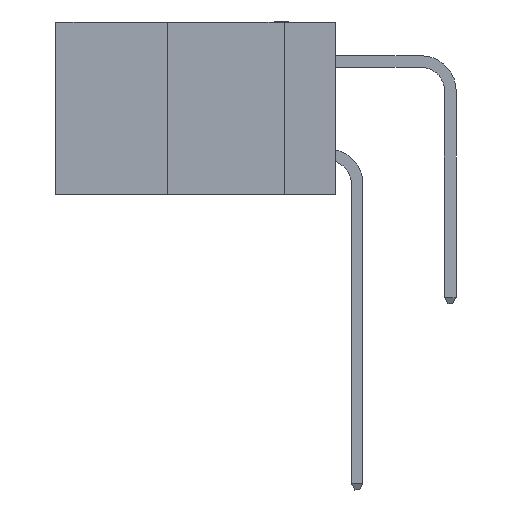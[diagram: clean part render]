
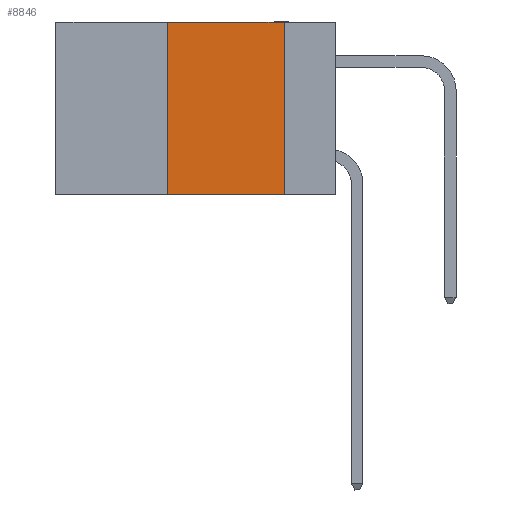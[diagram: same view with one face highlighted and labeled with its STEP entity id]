
A CAD part, left-side view. The second image highlights one B-rep face of the part: STEP entity #8846.
In plain terms, the highlighted planar face has unit normal (-1, 0, 0).
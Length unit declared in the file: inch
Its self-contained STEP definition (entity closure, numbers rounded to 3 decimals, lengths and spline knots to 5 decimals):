
#2086 = DIRECTION ( 'NONE',  ( 0., 0., -1. ) ) ;
#2624 = DIRECTION ( 'NONE',  ( 0., -1., 0. ) ) ;
#2887 = CARTESIAN_POINT ( 'NONE',  ( 0., 0.11, 0. ) ) ;
#3081 = VERTEX_POINT ( 'NONE', #8731 ) ;
#3131 = VECTOR ( 'NONE', #20635, 39.37008 ) ;
#3666 = ORIENTED_EDGE ( 'NONE', *, *, #10331, .F. ) ;
#5319 = ORIENTED_EDGE ( 'NONE', *, *, #9686, .T. ) ;
#6051 = CARTESIAN_POINT ( 'NONE',  ( 0., 0.6, -0.37 ) ) ;
#6799 = CARTESIAN_POINT ( 'NONE',  ( 0., 0.36, 0. ) ) ;
#7475 = DIRECTION ( 'NONE',  ( 0., 0., 1. ) ) ;
#8731 = CARTESIAN_POINT ( 'NONE',  ( 0., 0.11, 0. ) ) ;
#8846 = ADVANCED_FACE ( 'NONE', ( #18872 ), #16088, .F. ) ;
#9374 = LINE ( 'NONE', #6051, #3131 ) ;
#9686 = EDGE_CURVE ( 'NONE', #26777, #34970, #9374, .T. ) ;
#10331 = EDGE_CURVE ( 'NONE', #23102, #3081, #29275, .T. ) ;
#10421 = CARTESIAN_POINT ( 'NONE',  ( 0., 0.36, 0. ) ) ;
#10741 = DIRECTION ( 'NONE',  ( 1., 0., 0. ) ) ;
#13022 = CARTESIAN_POINT ( 'NONE',  ( 0., 0.36, -0.37 ) ) ;
#13854 = CARTESIAN_POINT ( 'NONE',  ( 0., 0.11, -0.37 ) ) ;
#16088 = PLANE ( 'NONE',  #21588 ) ;
#16873 = EDGE_LOOP ( 'NONE', ( #29009, #3666, #35339, #5319 ) ) ;
#18308 = EDGE_CURVE ( 'NONE', #26777, #23102, #31670, .T. ) ;
#18872 = FACE_OUTER_BOUND ( 'NONE', #16873, .T. ) ;
#19139 = VECTOR ( 'NONE', #2624, 39.37008 ) ;
#20635 = DIRECTION ( 'NONE',  ( 0., -1., 0. ) ) ;
#21588 = AXIS2_PLACEMENT_3D ( 'NONE', #27372, #10741, #2086 ) ;
#21931 = EDGE_CURVE ( 'NONE', #3081, #34970, #30224, .T. ) ;
#22438 = DIRECTION ( 'NONE',  ( 0., 0., -1. ) ) ;
#22921 = CARTESIAN_POINT ( 'NONE',  ( 0., 0.6, 0. ) ) ;
#23102 = VERTEX_POINT ( 'NONE', #6799 ) ;
#26744 = VECTOR ( 'NONE', #7475, 39.37008 ) ;
#26777 = VERTEX_POINT ( 'NONE', #13022 ) ;
#27372 = CARTESIAN_POINT ( 'NONE',  ( 0., 0.6, 0. ) ) ;
#29009 = ORIENTED_EDGE ( 'NONE', *, *, #21931, .F. ) ;
#29275 = LINE ( 'NONE', #22921, #19139 ) ;
#30224 = LINE ( 'NONE', #2887, #33942 ) ;
#31670 = LINE ( 'NONE', #10421, #26744 ) ;
#33942 = VECTOR ( 'NONE', #22438, 39.37008 ) ;
#34970 = VERTEX_POINT ( 'NONE', #13854 ) ;
#35339 = ORIENTED_EDGE ( 'NONE', *, *, #18308, .F. ) ;
